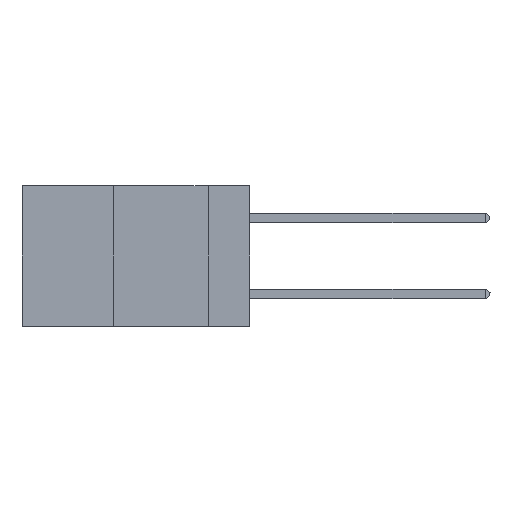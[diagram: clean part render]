
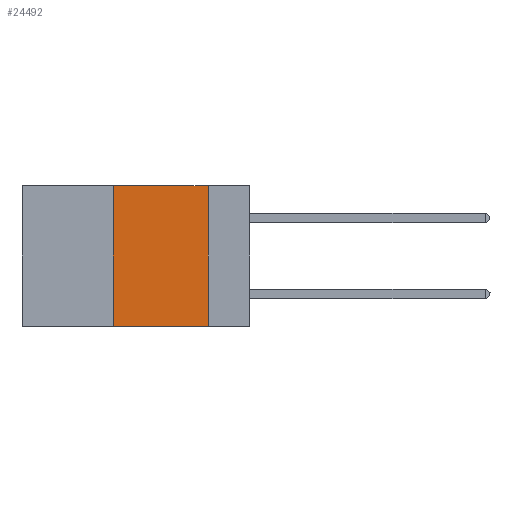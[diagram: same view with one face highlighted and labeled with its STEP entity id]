
A CAD part, left-side view. The second image highlights one B-rep face of the part: STEP entity #24492.
In plain terms, the highlighted planar face has unit normal (-1, 0, 0).
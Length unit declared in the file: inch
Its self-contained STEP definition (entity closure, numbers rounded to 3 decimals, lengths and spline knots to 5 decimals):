
#201 = VECTOR ( 'NONE', #18110, 39.37008 ) ;
#274 = AXIS2_PLACEMENT_3D ( 'NONE', #10798, #18650, #10877 ) ;
#962 = DIRECTION ( 'NONE',  ( 0., -1., 0. ) ) ;
#980 = VERTEX_POINT ( 'NONE', #23533 ) ;
#2718 = LINE ( 'NONE', #16753, #24809 ) ;
#4154 = LINE ( 'NONE', #13904, #22507 ) ;
#5167 = CARTESIAN_POINT ( 'NONE',  ( 0., 0.11, 0. ) ) ;
#5232 = CARTESIAN_POINT ( 'NONE',  ( 0., 0.11, -0.37 ) ) ;
#6257 = LINE ( 'NONE', #5167, #12686 ) ;
#6749 = FACE_OUTER_BOUND ( 'NONE', #24936, .T. ) ;
#7711 = VERTEX_POINT ( 'NONE', #5232 ) ;
#8599 = EDGE_CURVE ( 'NONE', #16351, #980, #4154, .T. ) ;
#9662 = LINE ( 'NONE', #24069, #201 ) ;
#10028 = CARTESIAN_POINT ( 'NONE',  ( 0., 0.11, 0. ) ) ;
#10798 = CARTESIAN_POINT ( 'NONE',  ( 0., 0.6, 0. ) ) ;
#10877 = DIRECTION ( 'NONE',  ( 0., 0., -1. ) ) ;
#12686 = VECTOR ( 'NONE', #14996, 39.37008 ) ;
#12898 = EDGE_CURVE ( 'NONE', #980, #16098, #2718, .T. ) ;
#13246 = DIRECTION ( 'NONE',  ( 0., 0., 1. ) ) ;
#13292 = CARTESIAN_POINT ( 'NONE',  ( 0., 0.36, -0.37 ) ) ;
#13904 = CARTESIAN_POINT ( 'NONE',  ( 0., 0.36, 0. ) ) ;
#14996 = DIRECTION ( 'NONE',  ( 0., 0., -1. ) ) ;
#16017 = ORIENTED_EDGE ( 'NONE', *, *, #22591, .T. ) ;
#16098 = VERTEX_POINT ( 'NONE', #10028 ) ;
#16351 = VERTEX_POINT ( 'NONE', #13292 ) ;
#16753 = CARTESIAN_POINT ( 'NONE',  ( 0., 0.6, 0. ) ) ;
#17289 = ORIENTED_EDGE ( 'NONE', *, *, #22213, .F. ) ;
#18110 = DIRECTION ( 'NONE',  ( 0., -1., 0. ) ) ;
#18650 = DIRECTION ( 'NONE',  ( 1., 0., 0. ) ) ;
#20370 = PLANE ( 'NONE',  #274 ) ;
#22213 = EDGE_CURVE ( 'NONE', #16098, #7711, #6257, .T. ) ;
#22507 = VECTOR ( 'NONE', #13246, 39.37008 ) ;
#22591 = EDGE_CURVE ( 'NONE', #16351, #7711, #9662, .T. ) ;
#23278 = ORIENTED_EDGE ( 'NONE', *, *, #12898, .F. ) ;
#23533 = CARTESIAN_POINT ( 'NONE',  ( 0., 0.36, 0. ) ) ;
#24069 = CARTESIAN_POINT ( 'NONE',  ( 0., 0.6, -0.37 ) ) ;
#24492 = ADVANCED_FACE ( 'NONE', ( #6749 ), #20370, .F. ) ;
#24809 = VECTOR ( 'NONE', #962, 39.37008 ) ;
#24936 = EDGE_LOOP ( 'NONE', ( #17289, #23278, #24956, #16017 ) ) ;
#24956 = ORIENTED_EDGE ( 'NONE', *, *, #8599, .F. ) ;
